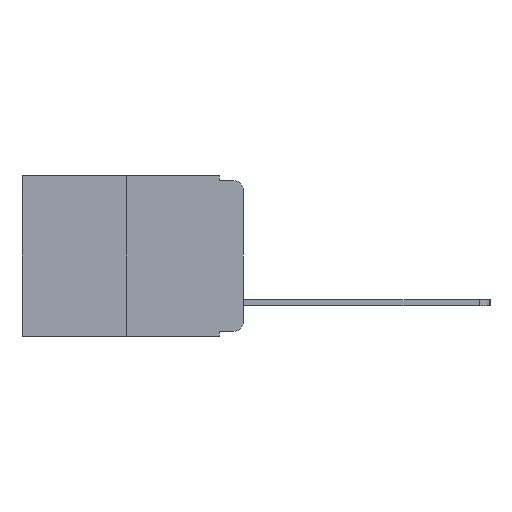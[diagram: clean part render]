
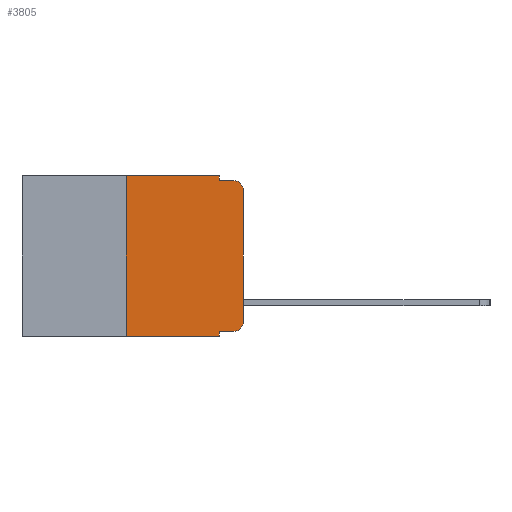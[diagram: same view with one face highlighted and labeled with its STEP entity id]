
A CAD part, left-side view. The second image highlights one B-rep face of the part: STEP entity #3805.
In plain terms, the highlighted planar face has unit normal (-1, 0, 0).
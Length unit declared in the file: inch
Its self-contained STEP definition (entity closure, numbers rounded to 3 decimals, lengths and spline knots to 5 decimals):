
#46 = CARTESIAN_POINT ( 'NONE',  ( 0., 0.25, -0.343 ) ) ;
#345 = ORIENTED_EDGE ( 'NONE', *, *, #4581, .F. ) ;
#352 = CARTESIAN_POINT ( 'NONE',  ( 0., 0.02, -0.03 ) ) ;
#523 = CARTESIAN_POINT ( 'NONE',  ( 0., 0.051, -0.333 ) ) ;
#828 = CARTESIAN_POINT ( 'NONE',  ( 0., 0.473, -0.343 ) ) ;
#1267 = DIRECTION ( 'NONE',  ( 0., 0., -1. ) ) ;
#1560 = ORIENTED_EDGE ( 'NONE', *, *, #2637, .F. ) ;
#1851 = DIRECTION ( 'NONE',  ( 0., 0., -1. ) ) ;
#1954 = VERTEX_POINT ( 'NONE', #46 ) ;
#2173 = CARTESIAN_POINT ( 'NONE',  ( 0., 0.051, -0.01 ) ) ;
#2324 = VERTEX_POINT ( 'NONE', #4093 ) ;
#2489 = CARTESIAN_POINT ( 'NONE',  ( 0., 0.051, -0.01 ) ) ;
#2637 = EDGE_CURVE ( 'NONE', #10886, #3828, #10179, .T. ) ;
#2695 = CARTESIAN_POINT ( 'NONE',  ( 0., 0.02, -0.313 ) ) ;
#2699 = LINE ( 'NONE', #16605, #10035 ) ;
#2842 = AXIS2_PLACEMENT_3D ( 'NONE', #2695, #12252, #4151 ) ;
#2909 = VERTEX_POINT ( 'NONE', #3149 ) ;
#3149 = CARTESIAN_POINT ( 'NONE',  ( 0., 0., -0.03 ) ) ;
#3526 = VERTEX_POINT ( 'NONE', #15575 ) ;
#3609 = DIRECTION ( 'NONE',  ( 0., 0., 1. ) ) ;
#3781 = AXIS2_PLACEMENT_3D ( 'NONE', #352, #10155, #1851 ) ;
#3805 = ADVANCED_FACE ( 'NONE', ( #7710 ), #6829, .F. ) ;
#3828 = VERTEX_POINT ( 'NONE', #7301 ) ;
#3836 = ORIENTED_EDGE ( 'NONE', *, *, #13813, .T. ) ;
#4011 = EDGE_LOOP ( 'NONE', ( #4760, #7405, #15260, #14670, #17284, #345, #16442, #1560, #7100, #3836 ) ) ;
#4093 = CARTESIAN_POINT ( 'NONE',  ( 0., 0.051, 0. ) ) ;
#4151 = DIRECTION ( 'NONE',  ( 0., 0., -1. ) ) ;
#4581 = EDGE_CURVE ( 'NONE', #1954, #7847, #10203, .T. ) ;
#4760 = ORIENTED_EDGE ( 'NONE', *, *, #16763, .T. ) ;
#5216 = CARTESIAN_POINT ( 'NONE',  ( 0., 0., 0. ) ) ;
#5579 = VECTOR ( 'NONE', #8065, 39.37008 ) ;
#5709 = VECTOR ( 'NONE', #1267, 39.37008 ) ;
#6350 = DIRECTION ( 'NONE',  ( 1., 0., 0. ) ) ;
#6624 = LINE ( 'NONE', #828, #9790 ) ;
#6829 = PLANE ( 'NONE',  #11769 ) ;
#7093 = LINE ( 'NONE', #8228, #17027 ) ;
#7095 = CIRCLE ( 'NONE', #2842, 0.02 ) ;
#7100 = ORIENTED_EDGE ( 'NONE', *, *, #12591, .T. ) ;
#7301 = CARTESIAN_POINT ( 'NONE',  ( 0., 0.051, -0.343 ) ) ;
#7405 = ORIENTED_EDGE ( 'NONE', *, *, #11651, .T. ) ;
#7536 = DIRECTION ( 'NONE',  ( 0., 0., -1. ) ) ;
#7710 = FACE_OUTER_BOUND ( 'NONE', #4011, .T. ) ;
#7847 = VERTEX_POINT ( 'NONE', #14003 ) ;
#8065 = DIRECTION ( 'NONE',  ( 0., -1., 0. ) ) ;
#8228 = CARTESIAN_POINT ( 'NONE',  ( 0., 0.473, 0. ) ) ;
#8349 = LINE ( 'NONE', #2173, #11491 ) ;
#8975 = CARTESIAN_POINT ( 'NONE',  ( 0., 0.25, 0. ) ) ;
#9352 = VECTOR ( 'NONE', #3609, 39.37008 ) ;
#9482 = EDGE_CURVE ( 'NONE', #2324, #9720, #2699, .T. ) ;
#9581 = EDGE_CURVE ( 'NONE', #9720, #15662, #8349, .T. ) ;
#9720 = VERTEX_POINT ( 'NONE', #2489 ) ;
#9790 = VECTOR ( 'NONE', #11887, 39.37008 ) ;
#9967 = VERTEX_POINT ( 'NONE', #15152 ) ;
#10035 = VECTOR ( 'NONE', #7536, 39.37008 ) ;
#10039 = LINE ( 'NONE', #12092, #5579 ) ;
#10155 = DIRECTION ( 'NONE',  ( -1., 0., 0. ) ) ;
#10179 = LINE ( 'NONE', #15008, #5709 ) ;
#10203 = LINE ( 'NONE', #8975, #9352 ) ;
#10707 = DIRECTION ( 'NONE',  ( 0., 0., 1. ) ) ;
#10886 = VERTEX_POINT ( 'NONE', #523 ) ;
#11196 = DIRECTION ( 'NONE',  ( 0., 0., -1. ) ) ;
#11313 = VECTOR ( 'NONE', #10707, 39.37008 ) ;
#11491 = VECTOR ( 'NONE', #13089, 39.37008 ) ;
#11651 = EDGE_CURVE ( 'NONE', #2909, #15662, #17281, .T. ) ;
#11769 = AXIS2_PLACEMENT_3D ( 'NONE', #16209, #6350, #11196 ) ;
#11887 = DIRECTION ( 'NONE',  ( 0., -1., 0. ) ) ;
#12092 = CARTESIAN_POINT ( 'NONE',  ( 0., 0.051, -0.333 ) ) ;
#12252 = DIRECTION ( 'NONE',  ( -1., 0., 0. ) ) ;
#12310 = DIRECTION ( 'NONE',  ( 0., -1., 0. ) ) ;
#12591 = EDGE_CURVE ( 'NONE', #10886, #9967, #10039, .T. ) ;
#13089 = DIRECTION ( 'NONE',  ( 0., -1., 0. ) ) ;
#13813 = EDGE_CURVE ( 'NONE', #9967, #3526, #7095, .T. ) ;
#14003 = CARTESIAN_POINT ( 'NONE',  ( 0., 0.25, 0. ) ) ;
#14259 = EDGE_CURVE ( 'NONE', #1954, #3828, #6624, .T. ) ;
#14670 = ORIENTED_EDGE ( 'NONE', *, *, #9482, .F. ) ;
#14740 = LINE ( 'NONE', #5216, #11313 ) ;
#15008 = CARTESIAN_POINT ( 'NONE',  ( 0., 0.051, 0. ) ) ;
#15152 = CARTESIAN_POINT ( 'NONE',  ( 0., 0.02, -0.333 ) ) ;
#15260 = ORIENTED_EDGE ( 'NONE', *, *, #9581, .F. ) ;
#15575 = CARTESIAN_POINT ( 'NONE',  ( 0., 0., -0.313 ) ) ;
#15662 = VERTEX_POINT ( 'NONE', #16916 ) ;
#16209 = CARTESIAN_POINT ( 'NONE',  ( 0., 0.473, 0. ) ) ;
#16442 = ORIENTED_EDGE ( 'NONE', *, *, #14259, .T. ) ;
#16605 = CARTESIAN_POINT ( 'NONE',  ( 0., 0.051, 0. ) ) ;
#16763 = EDGE_CURVE ( 'NONE', #3526, #2909, #14740, .T. ) ;
#16916 = CARTESIAN_POINT ( 'NONE',  ( 0., 0.02, -0.01 ) ) ;
#17027 = VECTOR ( 'NONE', #12310, 39.37008 ) ;
#17281 = CIRCLE ( 'NONE', #3781, 0.02 ) ;
#17284 = ORIENTED_EDGE ( 'NONE', *, *, #17389, .F. ) ;
#17389 = EDGE_CURVE ( 'NONE', #7847, #2324, #7093, .T. ) ;
